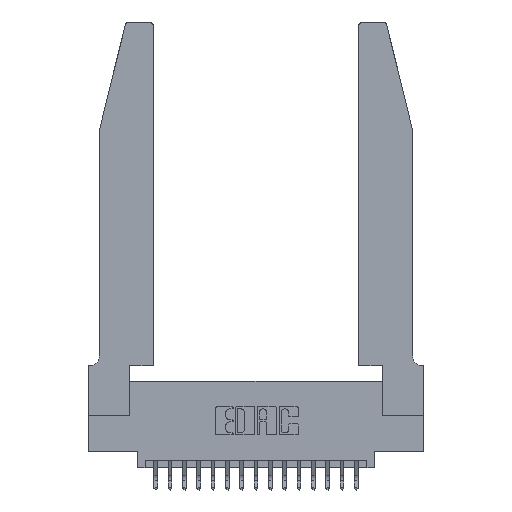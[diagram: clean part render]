
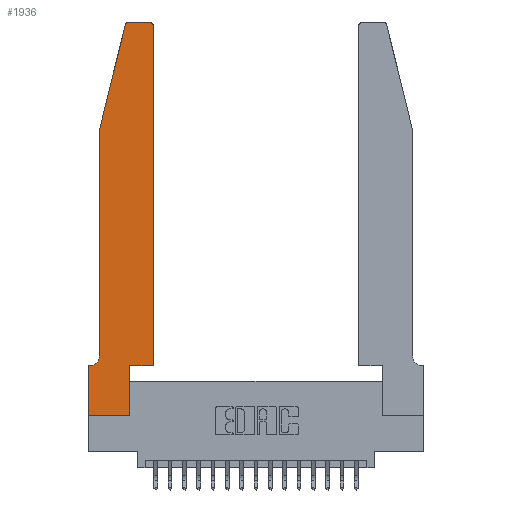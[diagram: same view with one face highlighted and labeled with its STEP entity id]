
A CAD part, top view. The second image highlights one B-rep face of the part: STEP entity #1936.
In plain terms, the highlighted planar face has unit normal (0, 0, 1).
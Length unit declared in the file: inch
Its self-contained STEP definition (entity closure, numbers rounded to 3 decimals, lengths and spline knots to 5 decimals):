
#101 = DIRECTION ( 'NONE',  ( 0., 0., -1. ) ) ;
#490 = LINE ( 'NONE', #1264, #9655 ) ;
#710 = VECTOR ( 'NONE', #11114, 39.37008 ) ;
#772 = ORIENTED_EDGE ( 'NONE', *, *, #4480, .T. ) ;
#798 = DIRECTION ( 'NONE',  ( -1., 0., 0. ) ) ;
#1014 = ORIENTED_EDGE ( 'NONE', *, *, #11486, .T. ) ;
#1264 = CARTESIAN_POINT ( 'NONE',  ( 0.4505, 0.35, 0.37 ) ) ;
#1756 = ORIENTED_EDGE ( 'NONE', *, *, #19671, .T. ) ;
#1936 = ADVANCED_FACE ( 'NONE', ( #11180 ), #17093, .T. ) ;
#2438 = DIRECTION ( 'NONE',  ( 0., 0., 1. ) ) ;
#2506 = CARTESIAN_POINT ( 'NONE',  ( 0.0755, 2., 0.37 ) ) ;
#2679 = CARTESIAN_POINT ( 'NONE',  ( 0.2865, 0., 0.37 ) ) ;
#2827 = LINE ( 'NONE', #2853, #10889 ) ;
#2842 = VERTEX_POINT ( 'NONE', #14744 ) ;
#2853 = CARTESIAN_POINT ( 'NONE',  ( 0.4505, 0.35, 0.37 ) ) ;
#2923 = DIRECTION ( 'NONE',  ( 1., 0., 0. ) ) ;
#2956 = LINE ( 'NONE', #2506, #6796 ) ;
#3088 = VERTEX_POINT ( 'NONE', #18581 ) ;
#3250 = VECTOR ( 'NONE', #798, 39.37008 ) ;
#3338 = AXIS2_PLACEMENT_3D ( 'NONE', #12081, #2438, #13644 ) ;
#3355 = VERTEX_POINT ( 'NONE', #11476 ) ;
#3433 = VERTEX_POINT ( 'NONE', #10118 ) ;
#3767 = EDGE_CURVE ( 'NONE', #17450, #7215, #490, .T. ) ;
#4480 = EDGE_CURVE ( 'NONE', #11318, #5929, #9386, .T. ) ;
#5020 = LINE ( 'NONE', #10361, #16196 ) ;
#5121 = ORIENTED_EDGE ( 'NONE', *, *, #16480, .T. ) ;
#5139 = AXIS2_PLACEMENT_3D ( 'NONE', #15985, #6515, #17543 ) ;
#5532 = EDGE_LOOP ( 'NONE', ( #772, #6317, #9268, #6718, #5121, #20032, #1014, #6710, #1756, #15958, #11020, #13891 ) ) ;
#5786 = CARTESIAN_POINT ( 'NONE',  ( 0.4505, 0.35, 0.37 ) ) ;
#5929 = VERTEX_POINT ( 'NONE', #14692 ) ;
#6045 = EDGE_CURVE ( 'NONE', #3355, #10532, #16200, .T. ) ;
#6161 = CARTESIAN_POINT ( 'NONE',  ( 0.0055, 0.35, 0.37 ) ) ;
#6317 = ORIENTED_EDGE ( 'NONE', *, *, #9621, .T. ) ;
#6411 = CARTESIAN_POINT ( 'NONE',  ( 0.0755, 0.42, 0.37 ) ) ;
#6515 = DIRECTION ( 'NONE',  ( 0., 0., 1. ) ) ;
#6710 = ORIENTED_EDGE ( 'NONE', *, *, #6045, .T. ) ;
#6718 = ORIENTED_EDGE ( 'NONE', *, *, #13606, .T. ) ;
#6796 = VECTOR ( 'NONE', #15305, 39.37008 ) ;
#7215 = VERTEX_POINT ( 'NONE', #16309 ) ;
#7864 = CARTESIAN_POINT ( 'NONE',  ( 0.2605, 2.75, 0.37 ) ) ;
#8640 = DIRECTION ( 'NONE',  ( 1., 0., 0. ) ) ;
#8858 = DIRECTION ( 'NONE',  ( 0., -1., 0. ) ) ;
#8933 = CARTESIAN_POINT ( 'NONE',  ( 0.0755, 0.35, 0.37 ) ) ;
#9265 = EDGE_CURVE ( 'NONE', #7215, #11318, #10650, .T. ) ;
#9268 = ORIENTED_EDGE ( 'NONE', *, *, #13685, .T. ) ;
#9386 = LINE ( 'NONE', #7864, #18170 ) ;
#9621 = EDGE_CURVE ( 'NONE', #5929, #10329, #14109, .T. ) ;
#9655 = VECTOR ( 'NONE', #10913, 39.37008 ) ;
#9837 = CARTESIAN_POINT ( 'NONE',  ( 0.0055, 0.42, 0.37 ) ) ;
#10021 = VERTEX_POINT ( 'NONE', #6161 ) ;
#10027 = EDGE_CURVE ( 'NONE', #2842, #17450, #2827, .T. ) ;
#10118 = CARTESIAN_POINT ( 'NONE',  ( 0.0755, 2., 0.37 ) ) ;
#10329 = VERTEX_POINT ( 'NONE', #19458 ) ;
#10361 = CARTESIAN_POINT ( 'NONE',  ( 0.0755, 2., 0.37 ) ) ;
#10476 = CARTESIAN_POINT ( 'NONE',  ( 0.2865, 0.35, 0.37 ) ) ;
#10532 = VERTEX_POINT ( 'NONE', #2679 ) ;
#10650 = CIRCLE ( 'NONE', #3338, 0.03 ) ;
#10682 = VERTEX_POINT ( 'NONE', #6411 ) ;
#10889 = VECTOR ( 'NONE', #2923, 39.37008 ) ;
#10913 = DIRECTION ( 'NONE',  ( 0., 1., 0. ) ) ;
#11020 = ORIENTED_EDGE ( 'NONE', *, *, #3767, .T. ) ;
#11068 = AXIS2_PLACEMENT_3D ( 'NONE', #17109, #17000, #16976 ) ;
#11114 = DIRECTION ( 'NONE',  ( 0., -1., 0. ) ) ;
#11180 = FACE_OUTER_BOUND ( 'NONE', #5532, .T. ) ;
#11318 = VERTEX_POINT ( 'NONE', #17411 ) ;
#11399 = DIRECTION ( 'NONE',  ( -1., 0., 0. ) ) ;
#11429 = CIRCLE ( 'NONE', #12051, 0.07 ) ;
#11476 = CARTESIAN_POINT ( 'NONE',  ( 0., 0., 0.37 ) ) ;
#11486 = EDGE_CURVE ( 'NONE', #3088, #3355, #17691, .T. ) ;
#11859 = EDGE_CURVE ( 'NONE', #10021, #3088, #20042, .T. ) ;
#12051 = AXIS2_PLACEMENT_3D ( 'NONE', #9837, #101, #11399 ) ;
#12061 = DIRECTION ( 'NONE',  ( 0., 1., 0. ) ) ;
#12081 = CARTESIAN_POINT ( 'NONE',  ( 0.4205, 2.72, 0.37 ) ) ;
#12497 = VECTOR ( 'NONE', #8640, 39.37008 ) ;
#13606 = EDGE_CURVE ( 'NONE', #3433, #10682, #5020, .T. ) ;
#13644 = DIRECTION ( 'NONE',  ( 1., 0., 0. ) ) ;
#13685 = EDGE_CURVE ( 'NONE', #10329, #3433, #2956, .T. ) ;
#13891 = ORIENTED_EDGE ( 'NONE', *, *, #9265, .T. ) ;
#14109 = CIRCLE ( 'NONE', #5139, 0.03 ) ;
#14692 = CARTESIAN_POINT ( 'NONE',  ( 0.284, 2.75, 0.37 ) ) ;
#14744 = CARTESIAN_POINT ( 'NONE',  ( 0.2865, 0.35, 0.37 ) ) ;
#15004 = LINE ( 'NONE', #10476, #19092 ) ;
#15305 = DIRECTION ( 'NONE',  ( -0.239, -0.971, 0. ) ) ;
#15958 = ORIENTED_EDGE ( 'NONE', *, *, #10027, .T. ) ;
#15985 = CARTESIAN_POINT ( 'NONE',  ( 0.284, 2.72, 0.37 ) ) ;
#16196 = VECTOR ( 'NONE', #8858, 39.37008 ) ;
#16200 = LINE ( 'NONE', #18012, #12497 ) ;
#16309 = CARTESIAN_POINT ( 'NONE',  ( 0.4505, 2.72, 0.37 ) ) ;
#16480 = EDGE_CURVE ( 'NONE', #10682, #10021, #11429, .T. ) ;
#16976 = DIRECTION ( 'NONE',  ( 1., 0., 0. ) ) ;
#17000 = DIRECTION ( 'NONE',  ( 0., 0., 1. ) ) ;
#17093 = PLANE ( 'NONE',  #11068 ) ;
#17109 = CARTESIAN_POINT ( 'NONE',  ( 0., 0.35, 0.37 ) ) ;
#17411 = CARTESIAN_POINT ( 'NONE',  ( 0.4205, 2.75, 0.37 ) ) ;
#17450 = VERTEX_POINT ( 'NONE', #5786 ) ;
#17543 = DIRECTION ( 'NONE',  ( 1., 0., 0. ) ) ;
#17691 = LINE ( 'NONE', #20385, #710 ) ;
#18012 = CARTESIAN_POINT ( 'NONE',  ( 0., 0., 0.37 ) ) ;
#18170 = VECTOR ( 'NONE', #18794, 39.37008 ) ;
#18581 = CARTESIAN_POINT ( 'NONE',  ( 0., 0.35, 0.37 ) ) ;
#18794 = DIRECTION ( 'NONE',  ( -1., 0., 0. ) ) ;
#19092 = VECTOR ( 'NONE', #12061, 39.37008 ) ;
#19458 = CARTESIAN_POINT ( 'NONE',  ( 0.25487, 2.72718, 0.37 ) ) ;
#19671 = EDGE_CURVE ( 'NONE', #10532, #2842, #15004, .T. ) ;
#20032 = ORIENTED_EDGE ( 'NONE', *, *, #11859, .T. ) ;
#20042 = LINE ( 'NONE', #8933, #3250 ) ;
#20385 = CARTESIAN_POINT ( 'NONE',  ( 0., 0., 0.37 ) ) ;
